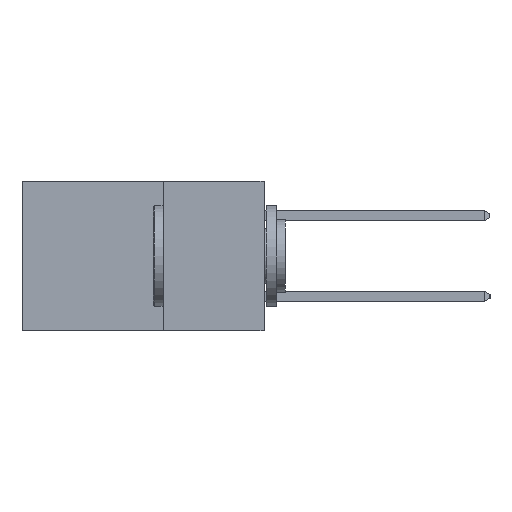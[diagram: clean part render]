
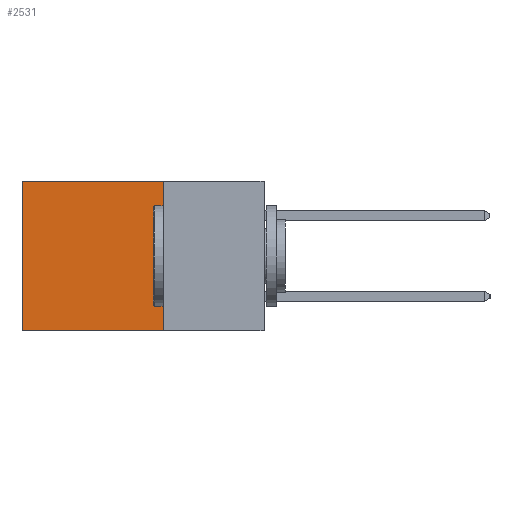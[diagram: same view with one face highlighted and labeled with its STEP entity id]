
A CAD part, left-side view. The second image highlights one B-rep face of the part: STEP entity #2531.
In plain terms, the highlighted planar face has unit normal (-1, 0, 0).
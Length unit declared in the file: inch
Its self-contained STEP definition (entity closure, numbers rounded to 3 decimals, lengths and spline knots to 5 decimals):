
#485 = VERTEX_POINT ( 'NONE', #14921 ) ;
#875 = LINE ( 'NONE', #7419, #5358 ) ;
#1118 = ORIENTED_EDGE ( 'NONE', *, *, #10022, .F. ) ;
#1256 = CARTESIAN_POINT ( 'NONE',  ( 0.2615, 0.6, -0.37 ) ) ;
#1290 = CARTESIAN_POINT ( 'NONE',  ( 0.2615, 0.25, -0.37 ) ) ;
#2525 = AXIS2_PLACEMENT_3D ( 'NONE', #10998, #10901, #7592 ) ;
#2531 = ADVANCED_FACE ( 'NONE', ( #17301 ), #10974, .F. ) ;
#3485 = DIRECTION ( 'NONE',  ( 0., 0., -1. ) ) ;
#4691 = LINE ( 'NONE', #12539, #12433 ) ;
#5358 = VECTOR ( 'NONE', #7170, 39.37008 ) ;
#6403 = VERTEX_POINT ( 'NONE', #1290 ) ;
#6673 = LINE ( 'NONE', #10737, #13913 ) ;
#7170 = DIRECTION ( 'NONE',  ( 0., 1., 0. ) ) ;
#7371 = EDGE_CURVE ( 'NONE', #6403, #11552, #875, .T. ) ;
#7419 = CARTESIAN_POINT ( 'NONE',  ( 0.2615, 0.25, -0.37 ) ) ;
#7592 = DIRECTION ( 'NONE',  ( 0., 0., -1. ) ) ;
#8626 = CARTESIAN_POINT ( 'NONE',  ( 0.2615, 0.25, 0. ) ) ;
#9647 = DIRECTION ( 'NONE',  ( 0., 0., -1. ) ) ;
#10022 = EDGE_CURVE ( 'NONE', #17521, #6403, #6673, .T. ) ;
#10100 = EDGE_CURVE ( 'NONE', #17521, #485, #16821, .T. ) ;
#10737 = CARTESIAN_POINT ( 'NONE',  ( 0.2615, 0.25, -0.37 ) ) ;
#10767 = ORIENTED_EDGE ( 'NONE', *, *, #13086, .T. ) ;
#10901 = DIRECTION ( 'NONE',  ( 1., 0., 0. ) ) ;
#10974 = PLANE ( 'NONE',  #2525 ) ;
#10998 = CARTESIAN_POINT ( 'NONE',  ( 0.2615, 0.25, -0.37 ) ) ;
#11026 = EDGE_LOOP ( 'NONE', ( #10767, #17085, #1118, #11076 ) ) ;
#11076 = ORIENTED_EDGE ( 'NONE', *, *, #10100, .T. ) ;
#11552 = VERTEX_POINT ( 'NONE', #1256 ) ;
#12433 = VECTOR ( 'NONE', #9647, 39.37008 ) ;
#12539 = CARTESIAN_POINT ( 'NONE',  ( 0.2615, 0.6, -0.37 ) ) ;
#12557 = VECTOR ( 'NONE', #16688, 39.37008 ) ;
#13086 = EDGE_CURVE ( 'NONE', #485, #11552, #4691, .T. ) ;
#13804 = CARTESIAN_POINT ( 'NONE',  ( 0.2615, 0.25, 0. ) ) ;
#13913 = VECTOR ( 'NONE', #3485, 39.37008 ) ;
#14921 = CARTESIAN_POINT ( 'NONE',  ( 0.2615, 0.6, 0. ) ) ;
#16688 = DIRECTION ( 'NONE',  ( 0., 1., 0. ) ) ;
#16821 = LINE ( 'NONE', #13804, #12557 ) ;
#17085 = ORIENTED_EDGE ( 'NONE', *, *, #7371, .F. ) ;
#17301 = FACE_OUTER_BOUND ( 'NONE', #11026, .T. ) ;
#17521 = VERTEX_POINT ( 'NONE', #8626 ) ;
